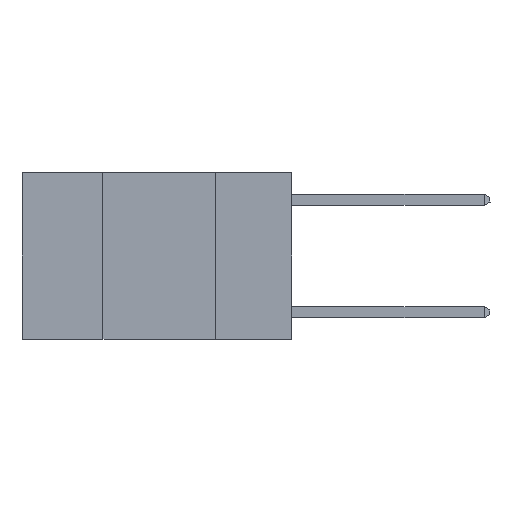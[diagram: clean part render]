
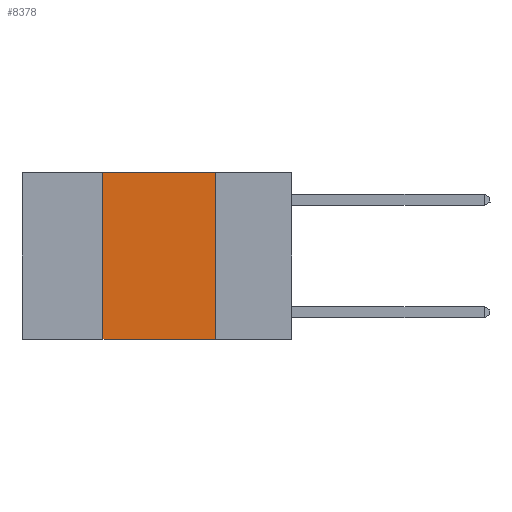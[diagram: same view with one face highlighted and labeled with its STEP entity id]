
A CAD part, left-side view. The second image highlights one B-rep face of the part: STEP entity #8378.
In plain terms, the highlighted planar face has unit normal (-1, 0, 0).
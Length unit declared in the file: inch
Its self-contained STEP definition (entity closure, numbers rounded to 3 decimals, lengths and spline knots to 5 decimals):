
#17 = CARTESIAN_POINT ( 'NONE',  ( 0., 0.42, -0.37 ) ) ;
#376 = DIRECTION ( 'NONE',  ( 1., 0., 0. ) ) ;
#1774 = LINE ( 'NONE', #2237, #5344 ) ;
#2237 = CARTESIAN_POINT ( 'NONE',  ( 0., 0.42, 0. ) ) ;
#2569 = CARTESIAN_POINT ( 'NONE',  ( 0., 0.6, 0. ) ) ;
#2647 = AXIS2_PLACEMENT_3D ( 'NONE', #4392, #376, #9614 ) ;
#4320 = CARTESIAN_POINT ( 'NONE',  ( 0., 0.17, 0. ) ) ;
#4392 = CARTESIAN_POINT ( 'NONE',  ( 0., 0.6, 0. ) ) ;
#4800 = VERTEX_POINT ( 'NONE', #8658 ) ;
#5344 = VECTOR ( 'NONE', #7562, 39.37008 ) ;
#5479 = VECTOR ( 'NONE', #12118, 39.37008 ) ;
#5864 = ORIENTED_EDGE ( 'NONE', *, *, #14410, .F. ) ;
#5892 = EDGE_CURVE ( 'NONE', #4800, #9230, #15328, .T. ) ;
#6001 = VECTOR ( 'NONE', #12914, 39.37008 ) ;
#6304 = LINE ( 'NONE', #14556, #5479 ) ;
#7407 = CARTESIAN_POINT ( 'NONE',  ( 0., 0.17, -0.37 ) ) ;
#7562 = DIRECTION ( 'NONE',  ( 0., 0., 1. ) ) ;
#7755 = VERTEX_POINT ( 'NONE', #14665 ) ;
#7978 = EDGE_CURVE ( 'NONE', #14513, #7755, #1774, .T. ) ;
#8301 = EDGE_LOOP ( 'NONE', ( #15568, #5864, #15171, #8935 ) ) ;
#8362 = PLANE ( 'NONE',  #2647 ) ;
#8378 = ADVANCED_FACE ( 'NONE', ( #15290 ), #8362, .F. ) ;
#8658 = CARTESIAN_POINT ( 'NONE',  ( 0., 0.17, 0. ) ) ;
#8935 = ORIENTED_EDGE ( 'NONE', *, *, #11356, .T. ) ;
#9230 = VERTEX_POINT ( 'NONE', #7407 ) ;
#9459 = VECTOR ( 'NONE', #13262, 39.37008 ) ;
#9614 = DIRECTION ( 'NONE',  ( 0., 0., -1. ) ) ;
#9817 = LINE ( 'NONE', #2569, #6001 ) ;
#11356 = EDGE_CURVE ( 'NONE', #14513, #9230, #6304, .T. ) ;
#12118 = DIRECTION ( 'NONE',  ( 0., -1., 0. ) ) ;
#12914 = DIRECTION ( 'NONE',  ( 0., -1., 0. ) ) ;
#13262 = DIRECTION ( 'NONE',  ( 0., 0., -1. ) ) ;
#14410 = EDGE_CURVE ( 'NONE', #7755, #4800, #9817, .T. ) ;
#14513 = VERTEX_POINT ( 'NONE', #17 ) ;
#14556 = CARTESIAN_POINT ( 'NONE',  ( 0., 0.6, -0.37 ) ) ;
#14665 = CARTESIAN_POINT ( 'NONE',  ( 0., 0.42, 0. ) ) ;
#15171 = ORIENTED_EDGE ( 'NONE', *, *, #7978, .F. ) ;
#15290 = FACE_OUTER_BOUND ( 'NONE', #8301, .T. ) ;
#15328 = LINE ( 'NONE', #4320, #9459 ) ;
#15568 = ORIENTED_EDGE ( 'NONE', *, *, #5892, .F. ) ;
